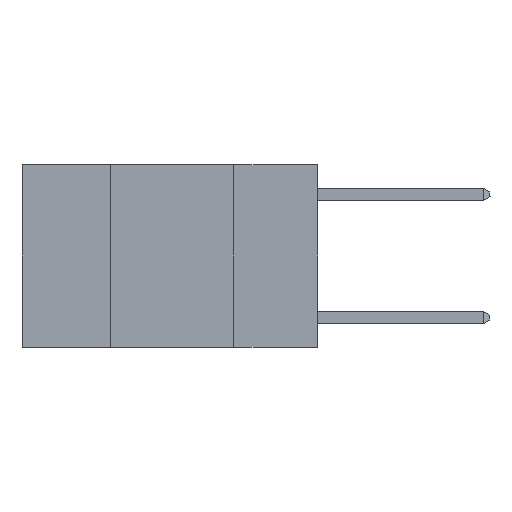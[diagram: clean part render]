
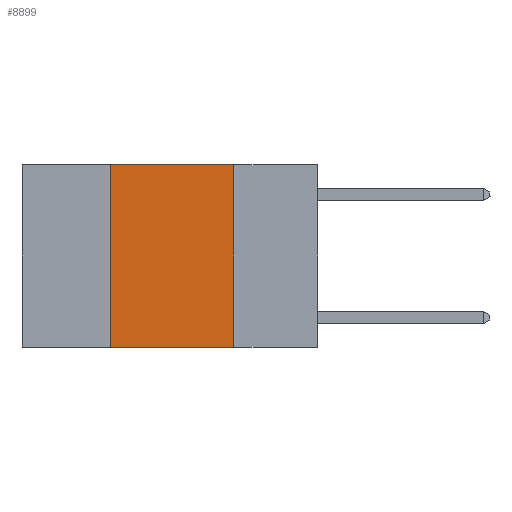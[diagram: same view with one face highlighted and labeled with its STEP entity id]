
A CAD part, left-side view. The second image highlights one B-rep face of the part: STEP entity #8899.
In plain terms, the highlighted planar face has unit normal (-1, 0, 0).
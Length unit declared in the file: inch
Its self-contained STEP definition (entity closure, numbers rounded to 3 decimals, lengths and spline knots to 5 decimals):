
#288 = DIRECTION ( 'NONE',  ( 0., -1., 0. ) ) ;
#459 = AXIS2_PLACEMENT_3D ( 'NONE', #6391, #584, #5733 ) ;
#584 = DIRECTION ( 'NONE',  ( 1., 0., 0. ) ) ;
#624 = FACE_OUTER_BOUND ( 'NONE', #3677, .T. ) ;
#872 = ORIENTED_EDGE ( 'NONE', *, *, #2548, .T. ) ;
#1109 = ORIENTED_EDGE ( 'NONE', *, *, #2382, .F. ) ;
#1393 = LINE ( 'NONE', #3315, #6915 ) ;
#1529 = VECTOR ( 'NONE', #7875, 39.37008 ) ;
#2032 = VERTEX_POINT ( 'NONE', #2335 ) ;
#2085 = CARTESIAN_POINT ( 'NONE',  ( 0., 0.17, 0. ) ) ;
#2335 = CARTESIAN_POINT ( 'NONE',  ( 0., 0.42, -0.37 ) ) ;
#2382 = EDGE_CURVE ( 'NONE', #3680, #4490, #9040, .T. ) ;
#2531 = EDGE_CURVE ( 'NONE', #2032, #5088, #1393, .T. ) ;
#2548 = EDGE_CURVE ( 'NONE', #2032, #4490, #3159, .T. ) ;
#3159 = LINE ( 'NONE', #8868, #6699 ) ;
#3315 = CARTESIAN_POINT ( 'NONE',  ( 0., 0.42, 0. ) ) ;
#3677 = EDGE_LOOP ( 'NONE', ( #1109, #4373, #8872, #872 ) ) ;
#3680 = VERTEX_POINT ( 'NONE', #2085 ) ;
#3866 = EDGE_CURVE ( 'NONE', #5088, #3680, #6664, .T. ) ;
#3921 = CARTESIAN_POINT ( 'NONE',  ( 0., 0.6, 0. ) ) ;
#4373 = ORIENTED_EDGE ( 'NONE', *, *, #3866, .F. ) ;
#4490 = VERTEX_POINT ( 'NONE', #7929 ) ;
#4905 = CARTESIAN_POINT ( 'NONE',  ( 0., 0.42, 0. ) ) ;
#5088 = VERTEX_POINT ( 'NONE', #4905 ) ;
#5733 = DIRECTION ( 'NONE',  ( 0., 0., -1. ) ) ;
#6014 = VECTOR ( 'NONE', #8040, 39.37008 ) ;
#6146 = DIRECTION ( 'NONE',  ( 0., 0., 1. ) ) ;
#6391 = CARTESIAN_POINT ( 'NONE',  ( 0., 0.6, 0. ) ) ;
#6664 = LINE ( 'NONE', #3921, #6014 ) ;
#6699 = VECTOR ( 'NONE', #288, 39.37008 ) ;
#6915 = VECTOR ( 'NONE', #6146, 39.37008 ) ;
#7875 = DIRECTION ( 'NONE',  ( 0., 0., -1. ) ) ;
#7929 = CARTESIAN_POINT ( 'NONE',  ( 0., 0.17, -0.37 ) ) ;
#8040 = DIRECTION ( 'NONE',  ( 0., -1., 0. ) ) ;
#8560 = CARTESIAN_POINT ( 'NONE',  ( 0., 0.17, 0. ) ) ;
#8868 = CARTESIAN_POINT ( 'NONE',  ( 0., 0.6, -0.37 ) ) ;
#8872 = ORIENTED_EDGE ( 'NONE', *, *, #2531, .F. ) ;
#8899 = ADVANCED_FACE ( 'NONE', ( #624 ), #9131, .F. ) ;
#9040 = LINE ( 'NONE', #8560, #1529 ) ;
#9131 = PLANE ( 'NONE',  #459 ) ;
